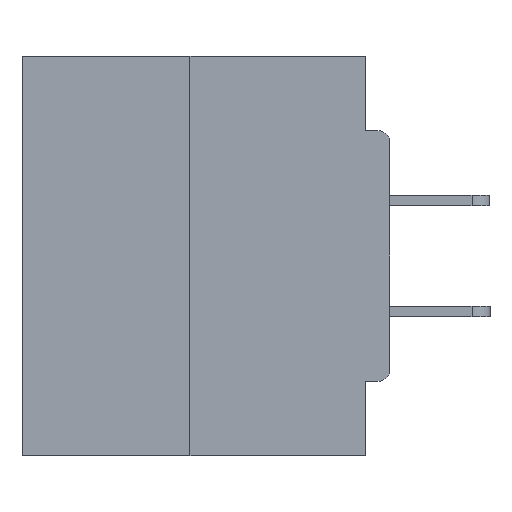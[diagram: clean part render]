
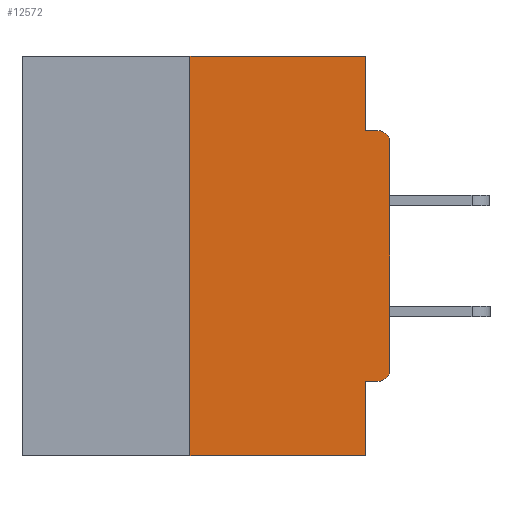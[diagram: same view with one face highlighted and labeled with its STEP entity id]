
A CAD part, left-side view. The second image highlights one B-rep face of the part: STEP entity #12572.
In plain terms, the highlighted planar face has unit normal (-1, 0, 0).
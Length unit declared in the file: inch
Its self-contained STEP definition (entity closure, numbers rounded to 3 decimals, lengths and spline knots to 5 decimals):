
#183 = EDGE_CURVE ( 'NONE', #2505, #2914, #31148, .T. ) ;
#366 = ORIENTED_EDGE ( 'NONE', *, *, #8094, .F. ) ;
#524 = AXIS2_PLACEMENT_3D ( 'NONE', #13885, #25160, #16476 ) ;
#665 = PLANE ( 'NONE',  #20704 ) ;
#1277 = VECTOR ( 'NONE', #16039, 39.37008 ) ;
#1732 = DIRECTION ( 'NONE',  ( 0., -1., 0. ) ) ;
#1805 = EDGE_CURVE ( 'NONE', #36528, #22187, #22144, .T. ) ;
#2120 = EDGE_LOOP ( 'NONE', ( #11059, #366, #22152, #35715, #9992, #10418, #4189, #25140, #15776, #16451 ) ) ;
#2505 = VERTEX_POINT ( 'NONE', #11500 ) ;
#2914 = VERTEX_POINT ( 'NONE', #19185 ) ;
#2935 = EDGE_CURVE ( 'NONE', #27561, #15646, #30989, .T. ) ;
#3344 = CARTESIAN_POINT ( 'NONE',  ( 0., 0.46, 0. ) ) ;
#3489 = EDGE_CURVE ( 'NONE', #17924, #2505, #29152, .T. ) ;
#4189 = ORIENTED_EDGE ( 'NONE', *, *, #2935, .T. ) ;
#4506 = CARTESIAN_POINT ( 'NONE',  ( 0., 0.25, 0. ) ) ;
#4764 = LINE ( 'NONE', #14153, #20738 ) ;
#4822 = DIRECTION ( 'NONE',  ( 0., 0., -1. ) ) ;
#7085 = DIRECTION ( 'NONE',  ( 0., 0., -1. ) ) ;
#8094 = EDGE_CURVE ( 'NONE', #18829, #28762, #11847, .T. ) ;
#8299 = CARTESIAN_POINT ( 'NONE',  ( 0., 0., -0.4065 ) ) ;
#9025 = VECTOR ( 'NONE', #1732, 39.37008 ) ;
#9903 = DIRECTION ( 'NONE',  ( 0., 0., 1. ) ) ;
#9992 = ORIENTED_EDGE ( 'NONE', *, *, #3489, .F. ) ;
#10196 = CARTESIAN_POINT ( 'NONE',  ( 0., 0., -0.3915 ) ) ;
#10292 = LINE ( 'NONE', #3344, #21004 ) ;
#10418 = ORIENTED_EDGE ( 'NONE', *, *, #19601, .T. ) ;
#11059 = ORIENTED_EDGE ( 'NONE', *, *, #17593, .F. ) ;
#11500 = CARTESIAN_POINT ( 'NONE',  ( 0., 0.031, -0.4065 ) ) ;
#11638 = CARTESIAN_POINT ( 'NONE',  ( 0., 0.015, -0.0935 ) ) ;
#11723 = AXIS2_PLACEMENT_3D ( 'NONE', #27342, #33046, #4822 ) ;
#11847 = LINE ( 'NONE', #4506, #31390 ) ;
#12572 = ADVANCED_FACE ( 'NONE', ( #17115 ), #665, .F. ) ;
#12954 = CARTESIAN_POINT ( 'NONE',  ( 0., 0., -0.0935 ) ) ;
#12985 = CARTESIAN_POINT ( 'NONE',  ( 0., 0.46, -0.5 ) ) ;
#13043 = LINE ( 'NONE', #12985, #9025 ) ;
#13106 = CIRCLE ( 'NONE', #524, 0.015 ) ;
#13885 = CARTESIAN_POINT ( 'NONE',  ( 0., 0.015, -0.1085 ) ) ;
#14060 = CARTESIAN_POINT ( 'NONE',  ( 0., 0.015, -0.4065 ) ) ;
#14153 = CARTESIAN_POINT ( 'NONE',  ( 0., 0.031, 0. ) ) ;
#14602 = VECTOR ( 'NONE', #24452, 39.37008 ) ;
#15646 = VERTEX_POINT ( 'NONE', #19665 ) ;
#15776 = ORIENTED_EDGE ( 'NONE', *, *, #1805, .F. ) ;
#16039 = DIRECTION ( 'NONE',  ( 0., 0., 1. ) ) ;
#16451 = ORIENTED_EDGE ( 'NONE', *, *, #17042, .F. ) ;
#16476 = DIRECTION ( 'NONE',  ( 0., 0., -1. ) ) ;
#17042 = EDGE_CURVE ( 'NONE', #32532, #36528, #4764, .T. ) ;
#17115 = FACE_OUTER_BOUND ( 'NONE', #2120, .T. ) ;
#17593 = EDGE_CURVE ( 'NONE', #28762, #32532, #10292, .T. ) ;
#17924 = VERTEX_POINT ( 'NONE', #14060 ) ;
#18098 = CARTESIAN_POINT ( 'NONE',  ( 0., 0.031, -0.5 ) ) ;
#18829 = VERTEX_POINT ( 'NONE', #26210 ) ;
#18959 = DIRECTION ( 'NONE',  ( 0., 0., -1. ) ) ;
#19135 = CIRCLE ( 'NONE', #11723, 0.015 ) ;
#19185 = CARTESIAN_POINT ( 'NONE',  ( 0., 0.031, -0.5 ) ) ;
#19601 = EDGE_CURVE ( 'NONE', #17924, #27561, #19135, .T. ) ;
#19665 = CARTESIAN_POINT ( 'NONE',  ( 0., 0., -0.1085 ) ) ;
#20001 = CARTESIAN_POINT ( 'NONE',  ( 0., 0.031, 0. ) ) ;
#20494 = CARTESIAN_POINT ( 'NONE',  ( 0., 0.46, 0. ) ) ;
#20704 = AXIS2_PLACEMENT_3D ( 'NONE', #20494, #35325, #7085 ) ;
#20738 = VECTOR ( 'NONE', #28770, 39.37008 ) ;
#21004 = VECTOR ( 'NONE', #26094, 39.37008 ) ;
#22144 = LINE ( 'NONE', #12954, #14602 ) ;
#22152 = ORIENTED_EDGE ( 'NONE', *, *, #23371, .T. ) ;
#22187 = VERTEX_POINT ( 'NONE', #11638 ) ;
#22572 = CARTESIAN_POINT ( 'NONE',  ( 0., 0.031, -0.0935 ) ) ;
#23371 = EDGE_CURVE ( 'NONE', #18829, #2914, #13043, .T. ) ;
#24452 = DIRECTION ( 'NONE',  ( 0., -1., 0. ) ) ;
#25140 = ORIENTED_EDGE ( 'NONE', *, *, #27151, .T. ) ;
#25160 = DIRECTION ( 'NONE',  ( -1., 0., 0. ) ) ;
#26094 = DIRECTION ( 'NONE',  ( 0., -1., 0. ) ) ;
#26210 = CARTESIAN_POINT ( 'NONE',  ( 0., 0.25, -0.5 ) ) ;
#27151 = EDGE_CURVE ( 'NONE', #15646, #22187, #13106, .T. ) ;
#27342 = CARTESIAN_POINT ( 'NONE',  ( 0., 0.015, -0.3915 ) ) ;
#27561 = VERTEX_POINT ( 'NONE', #10196 ) ;
#28762 = VERTEX_POINT ( 'NONE', #35450 ) ;
#28770 = DIRECTION ( 'NONE',  ( 0., 0., -1. ) ) ;
#29152 = LINE ( 'NONE', #8299, #35800 ) ;
#30989 = LINE ( 'NONE', #33277, #1277 ) ;
#31148 = LINE ( 'NONE', #18098, #33815 ) ;
#31390 = VECTOR ( 'NONE', #9903, 39.37008 ) ;
#32532 = VERTEX_POINT ( 'NONE', #20001 ) ;
#33046 = DIRECTION ( 'NONE',  ( -1., 0., 0. ) ) ;
#33277 = CARTESIAN_POINT ( 'NONE',  ( 0., 0., 0. ) ) ;
#33815 = VECTOR ( 'NONE', #18959, 39.37008 ) ;
#33844 = DIRECTION ( 'NONE',  ( 0., 1., 0. ) ) ;
#35325 = DIRECTION ( 'NONE',  ( 1., 0., 0. ) ) ;
#35450 = CARTESIAN_POINT ( 'NONE',  ( 0., 0.25, 0. ) ) ;
#35715 = ORIENTED_EDGE ( 'NONE', *, *, #183, .F. ) ;
#35800 = VECTOR ( 'NONE', #33844, 39.37008 ) ;
#36528 = VERTEX_POINT ( 'NONE', #22572 ) ;
